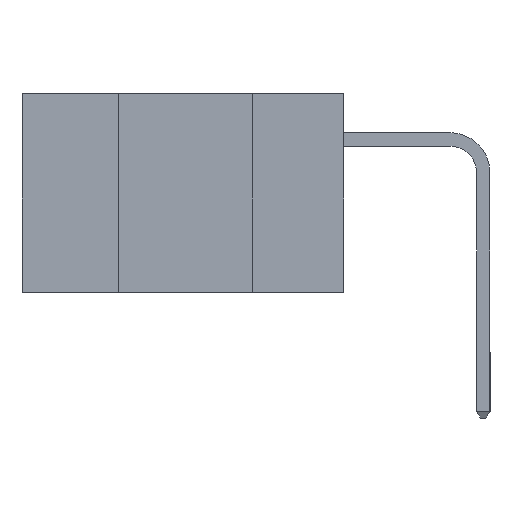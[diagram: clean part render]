
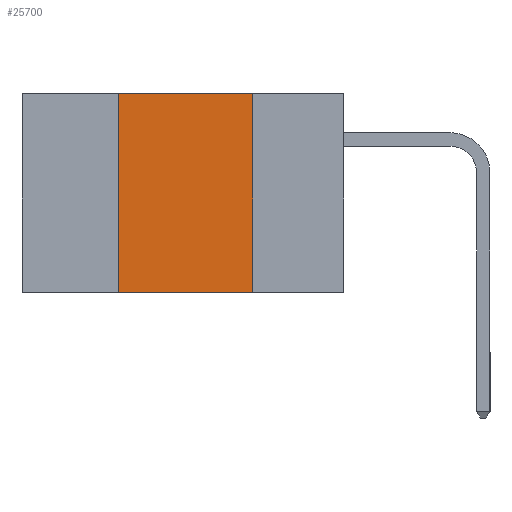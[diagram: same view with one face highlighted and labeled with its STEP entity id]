
A CAD part, left-side view. The second image highlights one B-rep face of the part: STEP entity #25700.
In plain terms, the highlighted planar face has unit normal (-1, 0, 0).
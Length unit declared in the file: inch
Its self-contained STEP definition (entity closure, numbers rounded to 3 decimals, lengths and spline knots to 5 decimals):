
#1087 = EDGE_CURVE ( 'NONE', #4179, #23833, #13614, .T. ) ;
#1710 = CARTESIAN_POINT ( 'NONE',  ( 0., 0.17, 0. ) ) ;
#2032 = LINE ( 'NONE', #8033, #21669 ) ;
#2088 = EDGE_CURVE ( 'NONE', #9435, #4179, #2032, .T. ) ;
#2659 = ORIENTED_EDGE ( 'NONE', *, *, #3953, .T. ) ;
#3953 = EDGE_CURVE ( 'NONE', #26317, #23833, #11335, .T. ) ;
#4179 = VERTEX_POINT ( 'NONE', #1710 ) ;
#5243 = ORIENTED_EDGE ( 'NONE', *, *, #2088, .F. ) ;
#6466 = CARTESIAN_POINT ( 'NONE',  ( 0., 0.42, -0.37 ) ) ;
#7055 = CARTESIAN_POINT ( 'NONE',  ( 0., 0.6, 0. ) ) ;
#8033 = CARTESIAN_POINT ( 'NONE',  ( 0., 0.6, 0. ) ) ;
#9435 = VERTEX_POINT ( 'NONE', #13251 ) ;
#9730 = DIRECTION ( 'NONE',  ( 0., 0., -1. ) ) ;
#10684 = CARTESIAN_POINT ( 'NONE',  ( 0., 0.17, -0.37 ) ) ;
#10931 = VECTOR ( 'NONE', #9730, 39.37008 ) ;
#11335 = LINE ( 'NONE', #15209, #19410 ) ;
#13058 = PLANE ( 'NONE',  #20329 ) ;
#13251 = CARTESIAN_POINT ( 'NONE',  ( 0., 0.42, 0. ) ) ;
#13614 = LINE ( 'NONE', #19911, #10931 ) ;
#14616 = LINE ( 'NONE', #6466, #22269 ) ;
#15209 = CARTESIAN_POINT ( 'NONE',  ( 0., 0.6, -0.37 ) ) ;
#16143 = EDGE_CURVE ( 'NONE', #26317, #9435, #14616, .T. ) ;
#18207 = ORIENTED_EDGE ( 'NONE', *, *, #1087, .F. ) ;
#19410 = VECTOR ( 'NONE', #19657, 39.37008 ) ;
#19514 = FACE_OUTER_BOUND ( 'NONE', #23188, .T. ) ;
#19657 = DIRECTION ( 'NONE',  ( 0., -1., 0. ) ) ;
#19740 = CARTESIAN_POINT ( 'NONE',  ( 0., 0.42, -0.37 ) ) ;
#19911 = CARTESIAN_POINT ( 'NONE',  ( 0., 0.17, -0.37 ) ) ;
#20329 = AXIS2_PLACEMENT_3D ( 'NONE', #7055, #21387, #23509 ) ;
#21387 = DIRECTION ( 'NONE',  ( 1., 0., 0. ) ) ;
#21669 = VECTOR ( 'NONE', #24474, 39.37008 ) ;
#22269 = VECTOR ( 'NONE', #22796, 39.37008 ) ;
#22796 = DIRECTION ( 'NONE',  ( 0., 0., 1. ) ) ;
#23188 = EDGE_LOOP ( 'NONE', ( #18207, #5243, #25636, #2659 ) ) ;
#23509 = DIRECTION ( 'NONE',  ( 0., 0., -1. ) ) ;
#23833 = VERTEX_POINT ( 'NONE', #10684 ) ;
#24474 = DIRECTION ( 'NONE',  ( 0., -1., 0. ) ) ;
#25636 = ORIENTED_EDGE ( 'NONE', *, *, #16143, .F. ) ;
#25700 = ADVANCED_FACE ( 'NONE', ( #19514 ), #13058, .F. ) ;
#26317 = VERTEX_POINT ( 'NONE', #19740 ) ;
